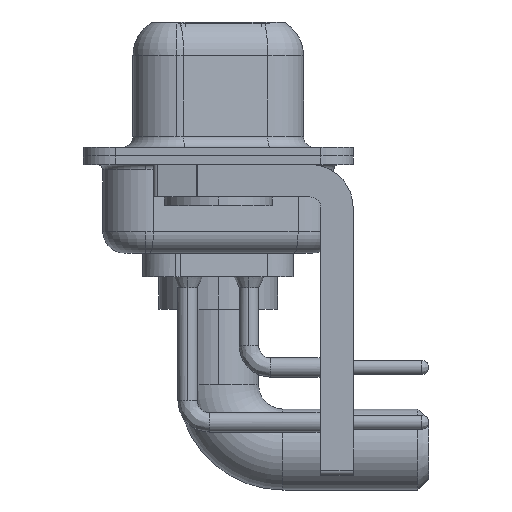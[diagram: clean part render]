
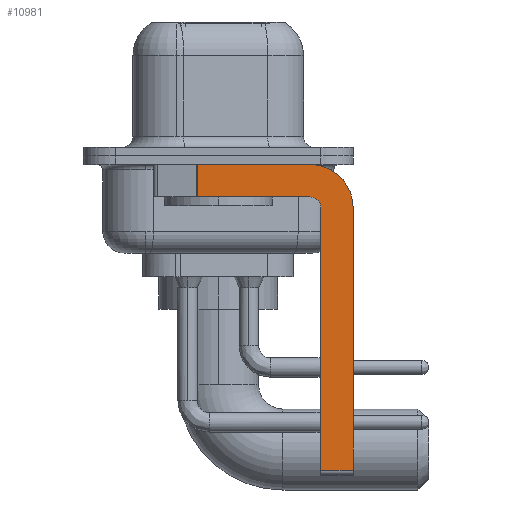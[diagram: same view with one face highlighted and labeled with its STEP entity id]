
A CAD part, left-side view. The second image highlights one B-rep face of the part: STEP entity #10981.
In plain terms, the highlighted planar face has unit normal (-1, 0, 0).
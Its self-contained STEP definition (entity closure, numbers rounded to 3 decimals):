
#312 = CIRCLE ( 'NONE', #16624, 2. ) ;
#715 = DIRECTION ( 'NONE',  ( 0., 0., -1. ) ) ;
#958 = CARTESIAN_POINT ( 'NONE',  ( -2.9, -6.25, -2.4 ) ) ;
#1376 = EDGE_CURVE ( 'NONE', #1739, #10512, #10575, .T. ) ;
#1422 = DIRECTION ( 'NONE',  ( 0., 0., -1. ) ) ;
#1739 = VERTEX_POINT ( 'NONE', #16737 ) ;
#1782 = DIRECTION ( 'NONE',  ( 1., 0., 0. ) ) ;
#2167 = CARTESIAN_POINT ( 'NONE',  ( -2.9, -6.25, -2.4 ) ) ;
#2325 = VECTOR ( 'NONE', #7383, 1000. ) ;
#3100 = LINE ( 'NONE', #958, #8783 ) ;
#3260 = VERTEX_POINT ( 'NONE', #19523 ) ;
#3294 = DIRECTION ( 'NONE',  ( 0., 0., 1. ) ) ;
#3696 = DIRECTION ( 'NONE',  ( 0., -1., 0. ) ) ;
#4827 = EDGE_CURVE ( 'NONE', #1739, #22479, #14635, .T. ) ;
#4936 = EDGE_CURVE ( 'NONE', #11996, #10781, #6051, .T. ) ;
#4975 = DIRECTION ( 'NONE',  ( -1., 0., 0. ) ) ;
#5116 = FACE_OUTER_BOUND ( 'NONE', #18964, .T. ) ;
#5352 = CARTESIAN_POINT ( 'NONE',  ( -2.9, -4.25, -1.9 ) ) ;
#6051 = LINE ( 'NONE', #17097, #8715 ) ;
#6494 = ORIENTED_EDGE ( 'NONE', *, *, #17965, .F. ) ;
#6510 = EDGE_CURVE ( 'NONE', #10512, #17213, #14497, .T. ) ;
#6537 = VECTOR ( 'NONE', #22535, 1000. ) ;
#7136 = LINE ( 'NONE', #5352, #2325 ) ;
#7383 = DIRECTION ( 'NONE',  ( 0., 1., 0. ) ) ;
#7506 = CARTESIAN_POINT ( 'NONE',  ( -2.9, -4.25, -1.9 ) ) ;
#8105 = CARTESIAN_POINT ( 'NONE',  ( -2.9, -6.25, -14.55 ) ) ;
#8715 = VECTOR ( 'NONE', #715, 1000. ) ;
#8783 = VECTOR ( 'NONE', #10354, 1000. ) ;
#8938 = CARTESIAN_POINT ( 'NONE',  ( -2.9, -4.75, -2.4 ) ) ;
#10268 = CARTESIAN_POINT ( 'NONE',  ( -2.9, 0.978, -0.4 ) ) ;
#10354 = DIRECTION ( 'NONE',  ( 0., 0., -1. ) ) ;
#10512 = VERTEX_POINT ( 'NONE', #8938 ) ;
#10564 = ORIENTED_EDGE ( 'NONE', *, *, #6510, .F. ) ;
#10575 = LINE ( 'NONE', #15901, #6537 ) ;
#10719 = VERTEX_POINT ( 'NONE', #2167 ) ;
#10781 = VERTEX_POINT ( 'NONE', #18857 ) ;
#10981 = ADVANCED_FACE ( 'NONE', ( #5116 ), #17784, .F. ) ;
#11332 = DIRECTION ( 'NONE',  ( 0., -1., 0. ) ) ;
#11861 = VECTOR ( 'NONE', #11332, 1000. ) ;
#11996 = VERTEX_POINT ( 'NONE', #10268 ) ;
#12146 = AXIS2_PLACEMENT_3D ( 'NONE', #18030, #1782, #1422 ) ;
#12221 = AXIS2_PLACEMENT_3D ( 'NONE', #16134, #4975, #3294 ) ;
#13172 = ORIENTED_EDGE ( 'NONE', *, *, #4827, .T. ) ;
#13227 = EDGE_CURVE ( 'NONE', #10719, #22479, #3100, .T. ) ;
#13412 = ORIENTED_EDGE ( 'NONE', *, *, #21321, .F. ) ;
#14330 = EDGE_CURVE ( 'NONE', #11996, #3260, #18653, .T. ) ;
#14497 = CIRCLE ( 'NONE', #12221, 0.5 ) ;
#14635 = LINE ( 'NONE', #21452, #19674 ) ;
#15019 = ORIENTED_EDGE ( 'NONE', *, *, #1376, .F. ) ;
#15649 = DIRECTION ( 'NONE',  ( 1., 0., 0. ) ) ;
#15901 = CARTESIAN_POINT ( 'NONE',  ( -2.9, -4.75, -14.8 ) ) ;
#16134 = CARTESIAN_POINT ( 'NONE',  ( -2.9, -4.25, -2.4 ) ) ;
#16624 = AXIS2_PLACEMENT_3D ( 'NONE', #20814, #15649, #22824 ) ;
#16737 = CARTESIAN_POINT ( 'NONE',  ( -2.9, -4.75, -14.55 ) ) ;
#16891 = CARTESIAN_POINT ( 'NONE',  ( -2.9, 3., -0.4 ) ) ;
#17097 = CARTESIAN_POINT ( 'NONE',  ( -2.9, 0.978, -1.9 ) ) ;
#17213 = VERTEX_POINT ( 'NONE', #7506 ) ;
#17784 = PLANE ( 'NONE',  #12146 ) ;
#17965 = EDGE_CURVE ( 'NONE', #3260, #10719, #312, .T. ) ;
#18030 = CARTESIAN_POINT ( 'NONE',  ( -2.9, -4.25, -2.4 ) ) ;
#18653 = LINE ( 'NONE', #16891, #11861 ) ;
#18857 = CARTESIAN_POINT ( 'NONE',  ( -2.9, 0.978, -1.9 ) ) ;
#18871 = ORIENTED_EDGE ( 'NONE', *, *, #14330, .F. ) ;
#18964 = EDGE_LOOP ( 'NONE', ( #18871, #21083, #13412, #10564, #15019, #13172, #23211, #6494 ) ) ;
#19523 = CARTESIAN_POINT ( 'NONE',  ( -2.9, -4.25, -0.4 ) ) ;
#19674 = VECTOR ( 'NONE', #3696, 1000. ) ;
#20814 = CARTESIAN_POINT ( 'NONE',  ( -2.9, -4.25, -2.4 ) ) ;
#21083 = ORIENTED_EDGE ( 'NONE', *, *, #4936, .T. ) ;
#21321 = EDGE_CURVE ( 'NONE', #17213, #10781, #7136, .T. ) ;
#21452 = CARTESIAN_POINT ( 'NONE',  ( -2.9, -4.25, -14.55 ) ) ;
#22479 = VERTEX_POINT ( 'NONE', #8105 ) ;
#22535 = DIRECTION ( 'NONE',  ( 0., 0., 1. ) ) ;
#22824 = DIRECTION ( 'NONE',  ( 0., 0., -1. ) ) ;
#23211 = ORIENTED_EDGE ( 'NONE', *, *, #13227, .F. ) ;
